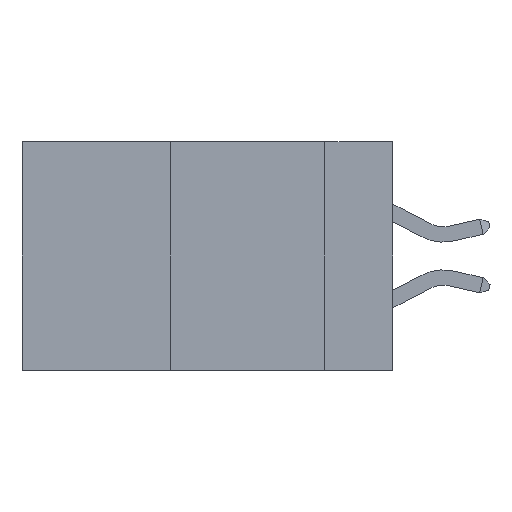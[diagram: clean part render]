
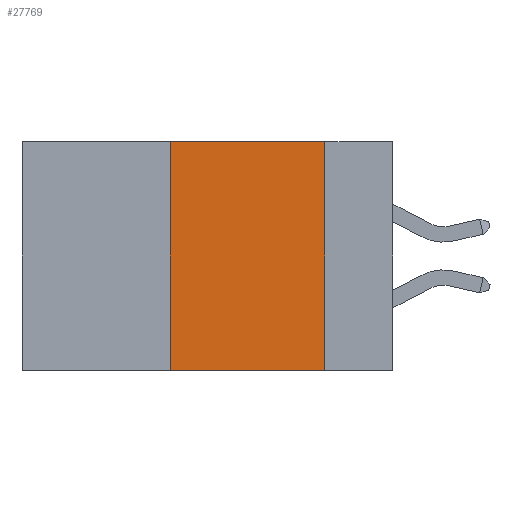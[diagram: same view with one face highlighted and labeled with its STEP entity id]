
A CAD part, left-side view. The second image highlights one B-rep face of the part: STEP entity #27769.
In plain terms, the highlighted planar face has unit normal (-1, 0, 0).
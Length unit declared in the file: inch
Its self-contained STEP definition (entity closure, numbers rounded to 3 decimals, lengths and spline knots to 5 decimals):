
#529 = LINE ( 'NONE', #1106, #24310 ) ;
#1106 = CARTESIAN_POINT ( 'NONE',  ( 0., 0.6, 0. ) ) ;
#1598 = DIRECTION ( 'NONE',  ( 0., 0., 1. ) ) ;
#1911 = EDGE_CURVE ( 'NONE', #24810, #13749, #28192, .T. ) ;
#3576 = LINE ( 'NONE', #6524, #28870 ) ;
#4757 = ORIENTED_EDGE ( 'NONE', *, *, #1911, .F. ) ;
#4770 = DIRECTION ( 'NONE',  ( 0., 0., -1. ) ) ;
#5083 = CARTESIAN_POINT ( 'NONE',  ( 0., 0.6, 0. ) ) ;
#6524 = CARTESIAN_POINT ( 'NONE',  ( 0., 0.36, 0. ) ) ;
#7263 = DIRECTION ( 'NONE',  ( 0., 0., -1. ) ) ;
#7670 = CARTESIAN_POINT ( 'NONE',  ( 0., 0.36, 0. ) ) ;
#7997 = VECTOR ( 'NONE', #7263, 39.37008 ) ;
#8257 = AXIS2_PLACEMENT_3D ( 'NONE', #5083, #9846, #4770 ) ;
#9597 = CARTESIAN_POINT ( 'NONE',  ( 0., 0.11, -0.37 ) ) ;
#9602 = CARTESIAN_POINT ( 'NONE',  ( 0., 0.11, 0. ) ) ;
#9846 = DIRECTION ( 'NONE',  ( 1., 0., 0. ) ) ;
#11031 = DIRECTION ( 'NONE',  ( 0., -1., 0. ) ) ;
#11107 = LINE ( 'NONE', #11648, #29695 ) ;
#11648 = CARTESIAN_POINT ( 'NONE',  ( 0., 0.6, -0.37 ) ) ;
#11669 = ORIENTED_EDGE ( 'NONE', *, *, #21388, .F. ) ;
#11802 = EDGE_LOOP ( 'NONE', ( #4757, #20144, #11669, #12218 ) ) ;
#11941 = VERTEX_POINT ( 'NONE', #15293 ) ;
#12218 = ORIENTED_EDGE ( 'NONE', *, *, #12940, .T. ) ;
#12940 = EDGE_CURVE ( 'NONE', #11941, #13749, #11107, .T. ) ;
#13749 = VERTEX_POINT ( 'NONE', #9597 ) ;
#15289 = PLANE ( 'NONE',  #8257 ) ;
#15293 = CARTESIAN_POINT ( 'NONE',  ( 0., 0.36, -0.37 ) ) ;
#20144 = ORIENTED_EDGE ( 'NONE', *, *, #25870, .F. ) ;
#21388 = EDGE_CURVE ( 'NONE', #11941, #30974, #3576, .T. ) ;
#24310 = VECTOR ( 'NONE', #11031, 39.37008 ) ;
#24810 = VERTEX_POINT ( 'NONE', #32175 ) ;
#25870 = EDGE_CURVE ( 'NONE', #30974, #24810, #529, .T. ) ;
#27769 = ADVANCED_FACE ( 'NONE', ( #27879 ), #15289, .F. ) ;
#27879 = FACE_OUTER_BOUND ( 'NONE', #11802, .T. ) ;
#28192 = LINE ( 'NONE', #9602, #7997 ) ;
#28870 = VECTOR ( 'NONE', #1598, 39.37008 ) ;
#29695 = VECTOR ( 'NONE', #31750, 39.37008 ) ;
#30974 = VERTEX_POINT ( 'NONE', #7670 ) ;
#31750 = DIRECTION ( 'NONE',  ( 0., -1., 0. ) ) ;
#32175 = CARTESIAN_POINT ( 'NONE',  ( 0., 0.11, 0. ) ) ;
